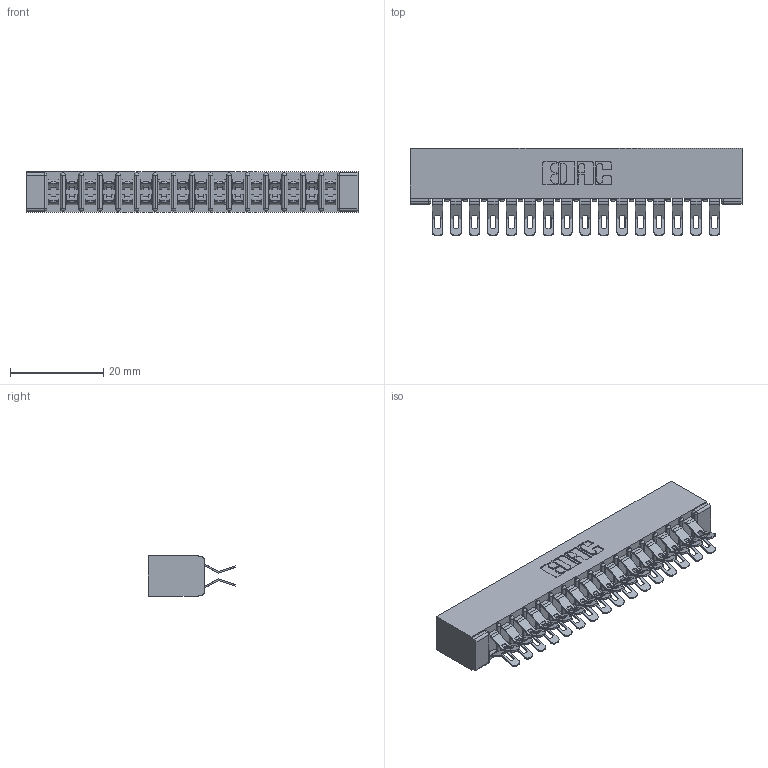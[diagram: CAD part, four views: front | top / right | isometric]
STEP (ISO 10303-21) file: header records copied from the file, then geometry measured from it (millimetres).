
FILE_DESCRIPTION (( 'STEP AP203' ), '1' );
FILE_NAME ('357-032-455-201.STEP', '2020-10-03T14:52:40', ( '' ), ( '' ), 'SwSTEP 2.0', 'SolidWorks 2020', '' );
FILE_SCHEMA (( 'CONFIG_CONTROL_DESIGN' ));
Length unit declared in the file: inch
Products named in the file (3): 307 Part_No Mounting Lugs; 357-032-455-201; 307-290-001_555
Assembly tree (33 placements, depth 2):
  357-032-455-201
    307 Part_No Mounting Lugs
    307-290-001_555  x32
Bounding box: 71.27 x 18.75 x 8.71 mm (x, y, z)
Volume: 4991.1 mm3; surface area: 9499.9 mm2
Topology: 33 solids, 33 shells, 2079 faces, 6091 edges, 3970 vertices
Faces by surface type: plane 1154, cylinder 891, sphere 34
Entity records: 17693 total; most frequent: CARTESIAN_POINT 2904, ORIENTED_EDGE 2876, DIRECTION 2862, EDGE_CURVE 1438, VECTOR 1082, LINE 1082, VERTEX_POINT 932, AXIS2_PLACEMENT_3D 890
